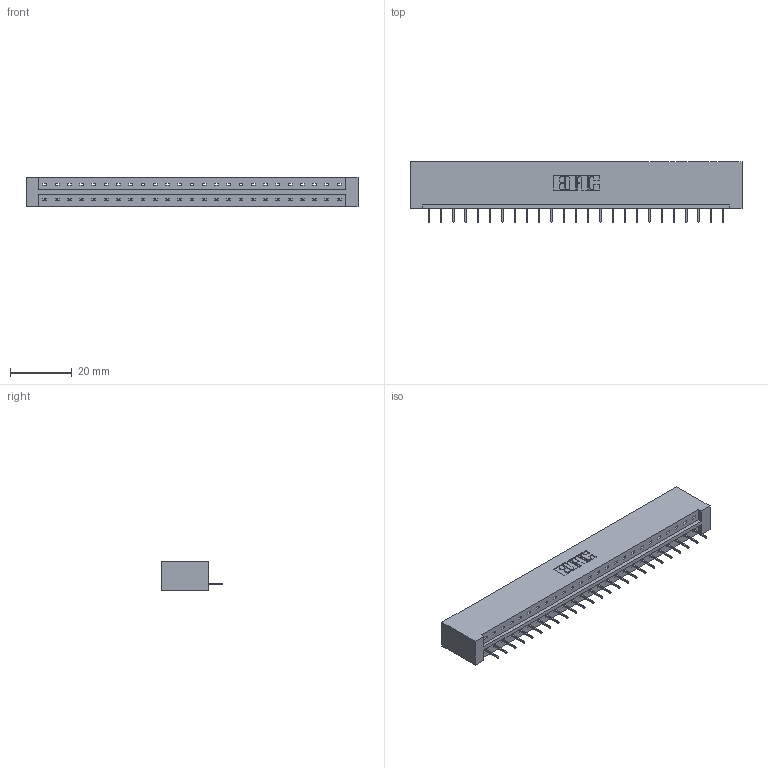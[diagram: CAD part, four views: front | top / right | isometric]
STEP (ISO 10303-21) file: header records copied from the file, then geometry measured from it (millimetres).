
FILE_DESCRIPTION (( 'STEP AP203' ), '1' );
FILE_NAME ('833-025-524-101.STEP', '2020-06-01T23:27:59', ( '' ), ( '' ), 'SwSTEP 2.0', 'SolidWorks 2020', '' );
FILE_SCHEMA (( 'CONFIG_CONTROL_DESIGN' ));
Length unit declared in the file: inch
Products named in the file (3): 345-292-001_345-293-124; 833-025-524-101; 833 Part_Lugless
Assembly tree (26 placements, depth 2):
  833-025-524-101
    833 Part_Lugless
    345-292-001_345-293-124  x25
Bounding box: 107.31 x 19.69 x 9.4 mm (x, y, z)
Volume: 11166.7 mm3; surface area: 11588 mm2
Topology: 26 solids, 26 shells, 1656 faces, 4787 edges, 3090 vertices
Faces by surface type: plane 1266, cylinder 390
Entity records: 17279 total; most frequent: CARTESIAN_POINT 2989, ORIENTED_EDGE 2950, DIRECTION 2549, EDGE_CURVE 1475, LINE 1359, VECTOR 1359, VERTEX_POINT 978, AXIS2_PLACEMENT_3D 595
